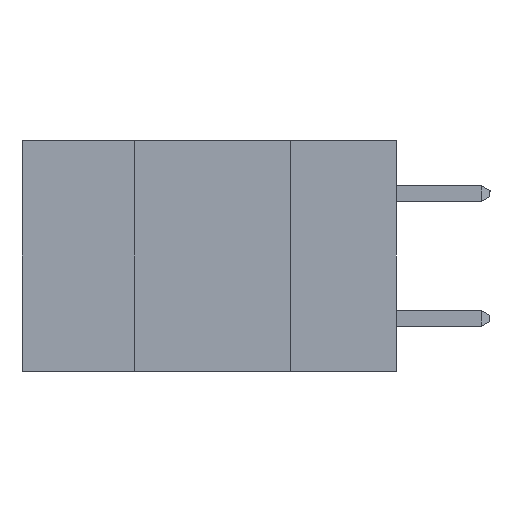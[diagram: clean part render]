
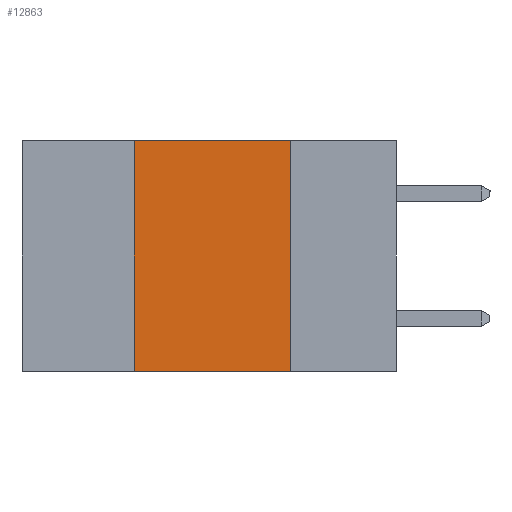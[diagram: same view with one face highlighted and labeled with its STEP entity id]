
A CAD part, left-side view. The second image highlights one B-rep face of the part: STEP entity #12863.
In plain terms, the highlighted planar face has unit normal (-1, 0, 0).
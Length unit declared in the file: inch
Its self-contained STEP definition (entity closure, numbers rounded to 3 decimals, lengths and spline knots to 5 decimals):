
#387 = CARTESIAN_POINT ( 'NONE',  ( 0., 0.17, -0.37 ) ) ;
#838 = VECTOR ( 'NONE', #1276, 39.37008 ) ;
#1276 = DIRECTION ( 'NONE',  ( 0., -1., 0. ) ) ;
#1907 = DIRECTION ( 'NONE',  ( 0., 0., -1. ) ) ;
#1976 = CARTESIAN_POINT ( 'NONE',  ( 0., 0.42, 0. ) ) ;
#2265 = DIRECTION ( 'NONE',  ( 0., 0., -1. ) ) ;
#3036 = LINE ( 'NONE', #387, #10162 ) ;
#3485 = VECTOR ( 'NONE', #3610, 39.37008 ) ;
#3569 = PLANE ( 'NONE',  #14332 ) ;
#3610 = DIRECTION ( 'NONE',  ( 0., -1., 0. ) ) ;
#4740 = EDGE_CURVE ( 'NONE', #6416, #14357, #12303, .T. ) ;
#4998 = VERTEX_POINT ( 'NONE', #1976 ) ;
#6286 = CARTESIAN_POINT ( 'NONE',  ( 0., 0.6, -0.37 ) ) ;
#6416 = VERTEX_POINT ( 'NONE', #7070 ) ;
#7070 = CARTESIAN_POINT ( 'NONE',  ( 0., 0.42, -0.37 ) ) ;
#7150 = LINE ( 'NONE', #10648, #9806 ) ;
#7822 = EDGE_CURVE ( 'NONE', #6416, #4998, #7150, .T. ) ;
#8883 = CARTESIAN_POINT ( 'NONE',  ( 0., 0.6, 0. ) ) ;
#8888 = CARTESIAN_POINT ( 'NONE',  ( 0., 0.6, 0. ) ) ;
#9076 = EDGE_LOOP ( 'NONE', ( #11248, #11052, #11549, #9909 ) ) ;
#9312 = CARTESIAN_POINT ( 'NONE',  ( 0., 0.17, 0. ) ) ;
#9521 = VERTEX_POINT ( 'NONE', #9312 ) ;
#9564 = DIRECTION ( 'NONE',  ( 0., 0., 1. ) ) ;
#9806 = VECTOR ( 'NONE', #9564, 39.37008 ) ;
#9909 = ORIENTED_EDGE ( 'NONE', *, *, #4740, .T. ) ;
#10162 = VECTOR ( 'NONE', #1907, 39.37008 ) ;
#10648 = CARTESIAN_POINT ( 'NONE',  ( 0., 0.42, -0.37 ) ) ;
#10983 = FACE_OUTER_BOUND ( 'NONE', #9076, .T. ) ;
#11052 = ORIENTED_EDGE ( 'NONE', *, *, #11622, .F. ) ;
#11248 = ORIENTED_EDGE ( 'NONE', *, *, #11825, .F. ) ;
#11549 = ORIENTED_EDGE ( 'NONE', *, *, #7822, .F. ) ;
#11622 = EDGE_CURVE ( 'NONE', #4998, #9521, #13883, .T. ) ;
#11825 = EDGE_CURVE ( 'NONE', #9521, #14357, #3036, .T. ) ;
#12303 = LINE ( 'NONE', #6286, #3485 ) ;
#12863 = ADVANCED_FACE ( 'NONE', ( #10983 ), #3569, .F. ) ;
#13799 = DIRECTION ( 'NONE',  ( 1., 0., 0. ) ) ;
#13883 = LINE ( 'NONE', #8883, #838 ) ;
#13956 = CARTESIAN_POINT ( 'NONE',  ( 0., 0.17, -0.37 ) ) ;
#14332 = AXIS2_PLACEMENT_3D ( 'NONE', #8888, #13799, #2265 ) ;
#14357 = VERTEX_POINT ( 'NONE', #13956 ) ;
